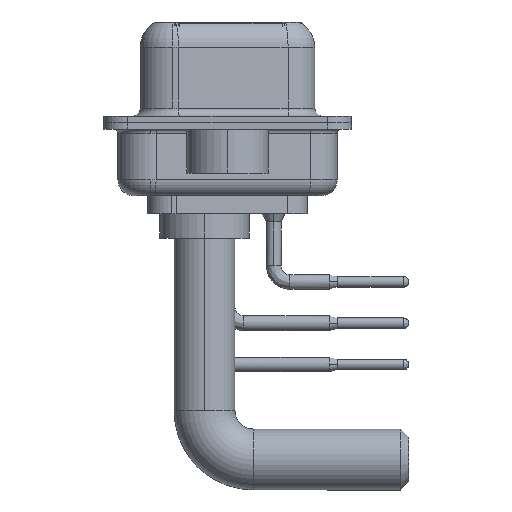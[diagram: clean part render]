
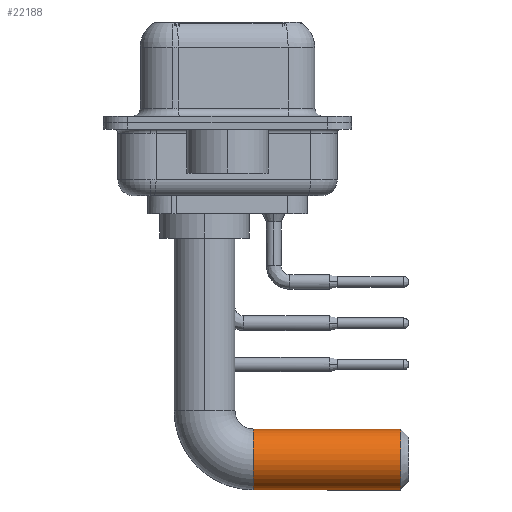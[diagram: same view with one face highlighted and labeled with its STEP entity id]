
A CAD part, left-side view. The second image highlights one B-rep face of the part: STEP entity #22188.
In plain terms, the highlighted cylindrical face has radius 1.875 mm (diameter 3.75 mm), a partial arc.
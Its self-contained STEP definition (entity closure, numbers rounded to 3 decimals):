
#387 = DIRECTION ( 'NONE',  ( 0., 0., -1. ) ) ;
#1082 = AXIS2_PLACEMENT_3D ( 'NONE', #11839, #14376, #387 ) ;
#1580 = DIRECTION ( 'NONE',  ( 0., -1., 0. ) ) ;
#1946 = VECTOR ( 'NONE', #17003, 1000. ) ;
#4066 = DIRECTION ( 'NONE',  ( 0., -1., 0. ) ) ;
#5130 = EDGE_LOOP ( 'NONE', ( #24741, #25911, #7584, #5989 ) ) ;
#5989 = ORIENTED_EDGE ( 'NONE', *, *, #11242, .T. ) ;
#6023 = CARTESIAN_POINT ( 'NONE',  ( 0., -3., -13.63 ) ) ;
#6630 = CARTESIAN_POINT ( 'NONE',  ( 0., -3., -11.755 ) ) ;
#7584 = ORIENTED_EDGE ( 'NONE', *, *, #8296, .T. ) ;
#8274 = DIRECTION ( 'NONE',  ( 0., 0., -1. ) ) ;
#8296 = EDGE_CURVE ( 'NONE', #9734, #27731, #21643, .T. ) ;
#8415 = FACE_OUTER_BOUND ( 'NONE', #5130, .T. ) ;
#8755 = EDGE_CURVE ( 'NONE', #27138, #13621, #10441, .T. ) ;
#9734 = VERTEX_POINT ( 'NONE', #19719 ) ;
#10006 = CARTESIAN_POINT ( 'NONE',  ( 0., -3., -13.63 ) ) ;
#10441 = LINE ( 'NONE', #19387, #1946 ) ;
#10700 = AXIS2_PLACEMENT_3D ( 'NONE', #6023, #1580, #8274 ) ;
#11242 = EDGE_CURVE ( 'NONE', #27731, #13621, #28149, .T. ) ;
#11476 = CIRCLE ( 'NONE', #12929, 1.875 ) ;
#11646 = CARTESIAN_POINT ( 'NONE',  ( 0., -12.07, -15.505 ) ) ;
#11839 = CARTESIAN_POINT ( 'NONE',  ( 0., -12.07, -13.63 ) ) ;
#12929 = AXIS2_PLACEMENT_3D ( 'NONE', #10006, #14319, #14762 ) ;
#13621 = VERTEX_POINT ( 'NONE', #19581 ) ;
#14319 = DIRECTION ( 'NONE',  ( 0., -1., 0. ) ) ;
#14376 = DIRECTION ( 'NONE',  ( 0., 1., 0. ) ) ;
#14762 = DIRECTION ( 'NONE',  ( -1., 0., 0. ) ) ;
#17003 = DIRECTION ( 'NONE',  ( 0., -1., 0. ) ) ;
#19167 = EDGE_CURVE ( 'NONE', #27138, #9734, #11476, .T. ) ;
#19387 = CARTESIAN_POINT ( 'NONE',  ( 0., -3., -11.755 ) ) ;
#19581 = CARTESIAN_POINT ( 'NONE',  ( 0., -12.07, -11.755 ) ) ;
#19592 = CYLINDRICAL_SURFACE ( 'NONE', #10700, 1.875 ) ;
#19719 = CARTESIAN_POINT ( 'NONE',  ( 0., -3., -15.505 ) ) ;
#21643 = LINE ( 'NONE', #28626, #28058 ) ;
#22188 = ADVANCED_FACE ( 'NONE', ( #8415 ), #19592, .T. ) ;
#24741 = ORIENTED_EDGE ( 'NONE', *, *, #8755, .F. ) ;
#25911 = ORIENTED_EDGE ( 'NONE', *, *, #19167, .T. ) ;
#27138 = VERTEX_POINT ( 'NONE', #6630 ) ;
#27731 = VERTEX_POINT ( 'NONE', #11646 ) ;
#28058 = VECTOR ( 'NONE', #4066, 1000. ) ;
#28149 = CIRCLE ( 'NONE', #1082, 1.875 ) ;
#28626 = CARTESIAN_POINT ( 'NONE',  ( 0., -3., -15.505 ) ) ;
